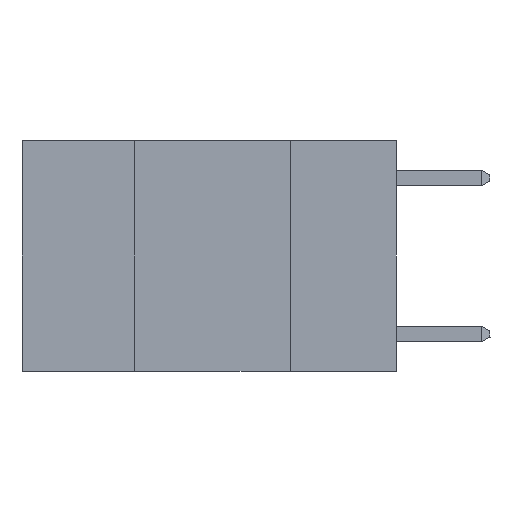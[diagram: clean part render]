
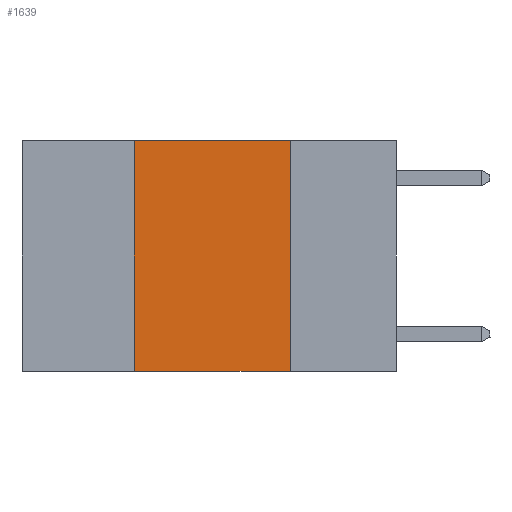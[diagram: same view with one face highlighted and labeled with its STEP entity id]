
A CAD part, left-side view. The second image highlights one B-rep face of the part: STEP entity #1639.
In plain terms, the highlighted planar face has unit normal (-1, 0, 0).
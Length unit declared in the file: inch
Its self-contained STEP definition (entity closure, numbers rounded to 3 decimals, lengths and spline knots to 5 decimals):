
#407 = DIRECTION ( 'NONE',  ( 0., 0., 1. ) ) ;
#479 = VERTEX_POINT ( 'NONE', #483 ) ;
#483 = CARTESIAN_POINT ( 'NONE',  ( 0., 0.42, 0. ) ) ;
#1008 = LINE ( 'NONE', #6057, #3570 ) ;
#1259 = ORIENTED_EDGE ( 'NONE', *, *, #3890, .F. ) ;
#1496 = VECTOR ( 'NONE', #3260, 39.37008 ) ;
#1501 = LINE ( 'NONE', #4137, #9759 ) ;
#1639 = ADVANCED_FACE ( 'NONE', ( #3635 ), #9709, .F. ) ;
#3170 = VERTEX_POINT ( 'NONE', #3915 ) ;
#3260 = DIRECTION ( 'NONE',  ( 0., -1., 0. ) ) ;
#3515 = CARTESIAN_POINT ( 'NONE',  ( 0., 0.17, 0. ) ) ;
#3570 = VECTOR ( 'NONE', #8233, 39.37008 ) ;
#3635 = FACE_OUTER_BOUND ( 'NONE', #7347, .T. ) ;
#3652 = LINE ( 'NONE', #7421, #5497 ) ;
#3890 = EDGE_CURVE ( 'NONE', #5362, #3170, #1008, .T. ) ;
#3915 = CARTESIAN_POINT ( 'NONE',  ( 0., 0.17, -0.37 ) ) ;
#4137 = CARTESIAN_POINT ( 'NONE',  ( 0., 0.42, 0. ) ) ;
#4235 = EDGE_CURVE ( 'NONE', #8423, #3170, #7490, .T. ) ;
#4824 = CARTESIAN_POINT ( 'NONE',  ( 0., 0.6, 0. ) ) ;
#5196 = EDGE_CURVE ( 'NONE', #8423, #479, #1501, .T. ) ;
#5362 = VERTEX_POINT ( 'NONE', #3515 ) ;
#5497 = VECTOR ( 'NONE', #6688, 39.37008 ) ;
#5618 = CARTESIAN_POINT ( 'NONE',  ( 0., 0.6, -0.37 ) ) ;
#5890 = CARTESIAN_POINT ( 'NONE',  ( 0., 0.42, -0.37 ) ) ;
#6057 = CARTESIAN_POINT ( 'NONE',  ( 0., 0.17, 0. ) ) ;
#6197 = AXIS2_PLACEMENT_3D ( 'NONE', #4824, #7209, #9220 ) ;
#6688 = DIRECTION ( 'NONE',  ( 0., -1., 0. ) ) ;
#7209 = DIRECTION ( 'NONE',  ( 1., 0., 0. ) ) ;
#7227 = ORIENTED_EDGE ( 'NONE', *, *, #4235, .T. ) ;
#7347 = EDGE_LOOP ( 'NONE', ( #1259, #8226, #10027, #7227 ) ) ;
#7421 = CARTESIAN_POINT ( 'NONE',  ( 0., 0.6, 0. ) ) ;
#7490 = LINE ( 'NONE', #5618, #1496 ) ;
#8226 = ORIENTED_EDGE ( 'NONE', *, *, #8509, .F. ) ;
#8233 = DIRECTION ( 'NONE',  ( 0., 0., -1. ) ) ;
#8423 = VERTEX_POINT ( 'NONE', #5890 ) ;
#8509 = EDGE_CURVE ( 'NONE', #479, #5362, #3652, .T. ) ;
#9220 = DIRECTION ( 'NONE',  ( 0., 0., -1. ) ) ;
#9709 = PLANE ( 'NONE',  #6197 ) ;
#9759 = VECTOR ( 'NONE', #407, 39.37008 ) ;
#10027 = ORIENTED_EDGE ( 'NONE', *, *, #5196, .F. ) ;
